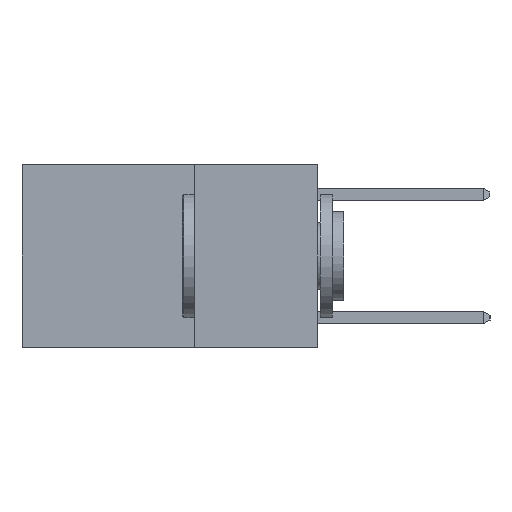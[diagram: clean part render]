
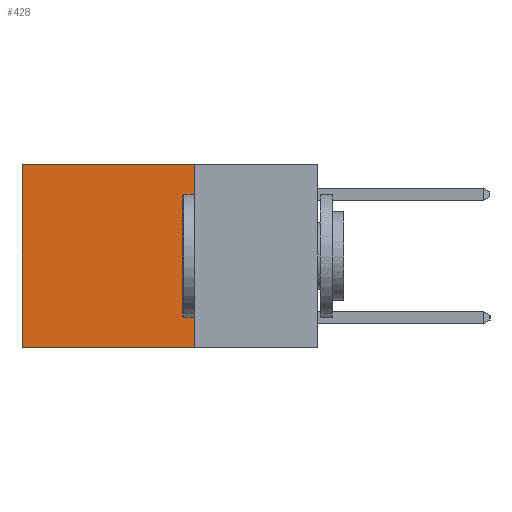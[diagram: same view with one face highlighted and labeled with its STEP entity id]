
A CAD part, left-side view. The second image highlights one B-rep face of the part: STEP entity #428.
In plain terms, the highlighted planar face has unit normal (-1, 0, 0).
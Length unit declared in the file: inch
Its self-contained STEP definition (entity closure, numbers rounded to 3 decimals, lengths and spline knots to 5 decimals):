
#13 = DIRECTION ( 'NONE',  ( 0., 0., -1. ) ) ;
#33 = EDGE_CURVE ( 'NONE', #614, #3680, #1793, .T. ) ;
#71 = ORIENTED_EDGE ( 'NONE', *, *, #5948, .F. ) ;
#428 = ADVANCED_FACE ( 'NONE', ( #8656 ), #5378, .F. ) ;
#550 = CARTESIAN_POINT ( 'NONE',  ( 0.2625, 0.25, 0. ) ) ;
#614 = VERTEX_POINT ( 'NONE', #1481 ) ;
#863 = CARTESIAN_POINT ( 'NONE',  ( 0.2625, 0.6, 0. ) ) ;
#1069 = DIRECTION ( 'NONE',  ( 0., 1., 0. ) ) ;
#1481 = CARTESIAN_POINT ( 'NONE',  ( 0.2625, 0.25, -0.37 ) ) ;
#1793 = LINE ( 'NONE', #3780, #6402 ) ;
#2300 = EDGE_LOOP ( 'NONE', ( #5790, #5999, #71, #6230 ) ) ;
#2851 = DIRECTION ( 'NONE',  ( 0., 1., 0. ) ) ;
#3008 = CARTESIAN_POINT ( 'NONE',  ( 0.2625, 0.25, 0. ) ) ;
#3079 = CARTESIAN_POINT ( 'NONE',  ( 0.2625, 0.6, -0.37 ) ) ;
#3680 = VERTEX_POINT ( 'NONE', #3079 ) ;
#3780 = CARTESIAN_POINT ( 'NONE',  ( 0.2625, 0.25, -0.37 ) ) ;
#4557 = VERTEX_POINT ( 'NONE', #550 ) ;
#5262 = DIRECTION ( 'NONE',  ( 0., 0., -1. ) ) ;
#5263 = DIRECTION ( 'NONE',  ( 0., 0., -1. ) ) ;
#5274 = DIRECTION ( 'NONE',  ( 1., 0., 0. ) ) ;
#5378 = PLANE ( 'NONE',  #7634 ) ;
#5570 = VECTOR ( 'NONE', #5262, 39.37008 ) ;
#5790 = ORIENTED_EDGE ( 'NONE', *, *, #9695, .T. ) ;
#5948 = EDGE_CURVE ( 'NONE', #4557, #614, #7801, .T. ) ;
#5977 = VERTEX_POINT ( 'NONE', #863 ) ;
#5999 = ORIENTED_EDGE ( 'NONE', *, *, #33, .F. ) ;
#6230 = ORIENTED_EDGE ( 'NONE', *, *, #9175, .T. ) ;
#6402 = VECTOR ( 'NONE', #2851, 39.37008 ) ;
#7359 = VECTOR ( 'NONE', #13, 39.37008 ) ;
#7630 = LINE ( 'NONE', #8657, #7359 ) ;
#7634 = AXIS2_PLACEMENT_3D ( 'NONE', #3008, #5274, #5263 ) ;
#7801 = LINE ( 'NONE', #11218, #5570 ) ;
#7957 = CARTESIAN_POINT ( 'NONE',  ( 0.2625, 0.25, 0. ) ) ;
#8465 = LINE ( 'NONE', #7957, #10455 ) ;
#8656 = FACE_OUTER_BOUND ( 'NONE', #2300, .T. ) ;
#8657 = CARTESIAN_POINT ( 'NONE',  ( 0.2625, 0.6, 0. ) ) ;
#9175 = EDGE_CURVE ( 'NONE', #4557, #5977, #8465, .T. ) ;
#9695 = EDGE_CURVE ( 'NONE', #5977, #3680, #7630, .T. ) ;
#10455 = VECTOR ( 'NONE', #1069, 39.37008 ) ;
#11218 = CARTESIAN_POINT ( 'NONE',  ( 0.2625, 0.25, 0. ) ) ;
